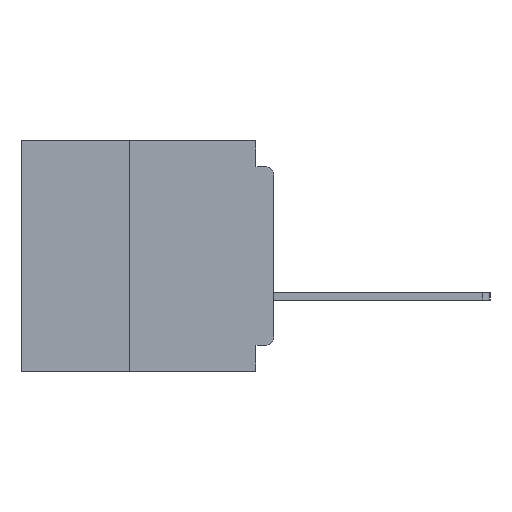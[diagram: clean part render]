
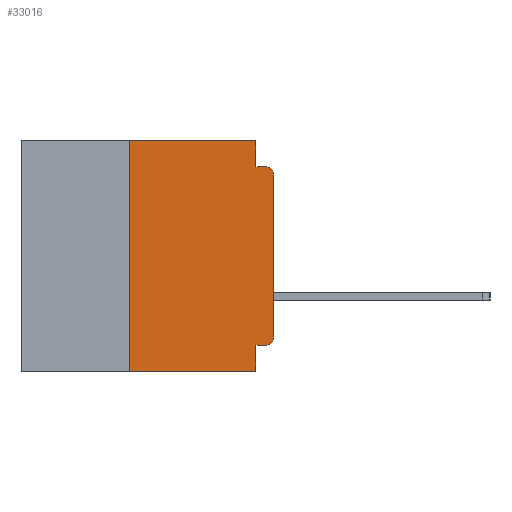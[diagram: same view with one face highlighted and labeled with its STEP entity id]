
A CAD part, left-side view. The second image highlights one B-rep face of the part: STEP entity #33016.
In plain terms, the highlighted planar face has unit normal (-1, 0, 0).
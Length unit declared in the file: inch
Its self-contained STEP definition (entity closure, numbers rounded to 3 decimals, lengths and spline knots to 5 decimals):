
#188 = LINE ( 'NONE', #37120, #32619 ) ;
#919 = CARTESIAN_POINT ( 'NONE',  ( 0., 0.031, 0. ) ) ;
#1937 = VECTOR ( 'NONE', #15777, 39.37008 ) ;
#7017 = LINE ( 'NONE', #22400, #28068 ) ;
#7413 = AXIS2_PLACEMENT_3D ( 'NONE', #40201, #14982, #44454 ) ;
#8552 = EDGE_CURVE ( 'NONE', #47240, #24752, #188, .T. ) ;
#8770 = DIRECTION ( 'NONE',  ( 0., 0., 1. ) ) ;
#9043 = CARTESIAN_POINT ( 'NONE',  ( 0., 0.25, -0.4 ) ) ;
#9058 = EDGE_CURVE ( 'NONE', #42572, #22171, #28692, .T. ) ;
#9689 = CARTESIAN_POINT ( 'NONE',  ( 0., 0.031, -0.355 ) ) ;
#11108 = ORIENTED_EDGE ( 'NONE', *, *, #8552, .T. ) ;
#11936 = ORIENTED_EDGE ( 'NONE', *, *, #54126, .T. ) ;
#12481 = VERTEX_POINT ( 'NONE', #44329 ) ;
#14232 = VERTEX_POINT ( 'NONE', #9689 ) ;
#14356 = DIRECTION ( 'NONE',  ( 0., -1., 0. ) ) ;
#14437 = DIRECTION ( 'NONE',  ( 0., 1., 0. ) ) ;
#14982 = DIRECTION ( 'NONE',  ( 1., 0., 0. ) ) ;
#15777 = DIRECTION ( 'NONE',  ( 0., -1., 0. ) ) ;
#17053 = VECTOR ( 'NONE', #14356, 39.37008 ) ;
#17242 = VERTEX_POINT ( 'NONE', #43105 ) ;
#17258 = CARTESIAN_POINT ( 'NONE',  ( 0., 0.015, -0.34 ) ) ;
#17575 = VECTOR ( 'NONE', #42715, 39.37008 ) ;
#18249 = DIRECTION ( 'NONE',  ( -1., 0., 0. ) ) ;
#18378 = CIRCLE ( 'NONE', #29910, 0.015 ) ;
#19150 = EDGE_CURVE ( 'NONE', #28937, #14232, #38069, .T. ) ;
#19928 = LINE ( 'NONE', #46576, #41058 ) ;
#21380 = EDGE_CURVE ( 'NONE', #14232, #12481, #7017, .T. ) ;
#21450 = DIRECTION ( 'NONE',  ( 0., 0., -1. ) ) ;
#22171 = VERTEX_POINT ( 'NONE', #53320 ) ;
#22198 = CARTESIAN_POINT ( 'NONE',  ( 0., 0., -0.34 ) ) ;
#22400 = CARTESIAN_POINT ( 'NONE',  ( 0., 0.031, -0.4 ) ) ;
#24056 = CARTESIAN_POINT ( 'NONE',  ( 0., 0.015, -0.045 ) ) ;
#24752 = VERTEX_POINT ( 'NONE', #25092 ) ;
#25092 = CARTESIAN_POINT ( 'NONE',  ( 0., 0., -0.06 ) ) ;
#25450 = VERTEX_POINT ( 'NONE', #9043 ) ;
#25738 = CIRCLE ( 'NONE', #34081, 0.015 ) ;
#26362 = ORIENTED_EDGE ( 'NONE', *, *, #49178, .F. ) ;
#27010 = EDGE_CURVE ( 'NONE', #25450, #12481, #27399, .T. ) ;
#27398 = VECTOR ( 'NONE', #36341, 39.37008 ) ;
#27399 = LINE ( 'NONE', #34395, #17575 ) ;
#27831 = CARTESIAN_POINT ( 'NONE',  ( 0., 0.031, 0. ) ) ;
#28068 = VECTOR ( 'NONE', #30875, 39.37008 ) ;
#28692 = LINE ( 'NONE', #27831, #27398 ) ;
#28937 = VERTEX_POINT ( 'NONE', #51762 ) ;
#29667 = EDGE_CURVE ( 'NONE', #28937, #47240, #25738, .T. ) ;
#29910 = AXIS2_PLACEMENT_3D ( 'NONE', #43495, #18249, #47762 ) ;
#30875 = DIRECTION ( 'NONE',  ( 0., 0., -1. ) ) ;
#32619 = VECTOR ( 'NONE', #53973, 39.37008 ) ;
#33016 = ADVANCED_FACE ( 'NONE', ( #48007 ), #35936, .F. ) ;
#33030 = LINE ( 'NONE', #41017, #1937 ) ;
#33533 = ORIENTED_EDGE ( 'NONE', *, *, #9058, .F. ) ;
#34081 = AXIS2_PLACEMENT_3D ( 'NONE', #17258, #46761, #21450 ) ;
#34160 = LINE ( 'NONE', #52342, #17053 ) ;
#34395 = CARTESIAN_POINT ( 'NONE',  ( 0., 0.437, -0.4 ) ) ;
#35936 = PLANE ( 'NONE',  #7413 ) ;
#36341 = DIRECTION ( 'NONE',  ( 0., 0., -1. ) ) ;
#36355 = VERTEX_POINT ( 'NONE', #24056 ) ;
#36379 = EDGE_LOOP ( 'NONE', ( #11108, #11936, #38645, #33533, #26362, #44519, #38637, #37073, #54459, #45050 ) ) ;
#36732 = VECTOR ( 'NONE', #14437, 39.37008 ) ;
#37073 = ORIENTED_EDGE ( 'NONE', *, *, #21380, .F. ) ;
#37120 = CARTESIAN_POINT ( 'NONE',  ( 0., 0., 0. ) ) ;
#38069 = LINE ( 'NONE', #39832, #36732 ) ;
#38637 = ORIENTED_EDGE ( 'NONE', *, *, #27010, .T. ) ;
#38645 = ORIENTED_EDGE ( 'NONE', *, *, #47443, .F. ) ;
#39832 = CARTESIAN_POINT ( 'NONE',  ( 0., 0., -0.355 ) ) ;
#40201 = CARTESIAN_POINT ( 'NONE',  ( 0., 0.437, 0. ) ) ;
#41017 = CARTESIAN_POINT ( 'NONE',  ( 0., 0., -0.045 ) ) ;
#41058 = VECTOR ( 'NONE', #8770, 39.37008 ) ;
#42572 = VERTEX_POINT ( 'NONE', #919 ) ;
#42715 = DIRECTION ( 'NONE',  ( 0., -1., 0. ) ) ;
#43105 = CARTESIAN_POINT ( 'NONE',  ( 0., 0.25, 0. ) ) ;
#43495 = CARTESIAN_POINT ( 'NONE',  ( 0., 0.015, -0.06 ) ) ;
#44033 = EDGE_CURVE ( 'NONE', #25450, #17242, #19928, .T. ) ;
#44329 = CARTESIAN_POINT ( 'NONE',  ( 0., 0.031, -0.4 ) ) ;
#44454 = DIRECTION ( 'NONE',  ( 0., 0., -1. ) ) ;
#44519 = ORIENTED_EDGE ( 'NONE', *, *, #44033, .F. ) ;
#45050 = ORIENTED_EDGE ( 'NONE', *, *, #29667, .T. ) ;
#46576 = CARTESIAN_POINT ( 'NONE',  ( 0., 0.25, -0.4 ) ) ;
#46761 = DIRECTION ( 'NONE',  ( -1., 0., 0. ) ) ;
#47240 = VERTEX_POINT ( 'NONE', #22198 ) ;
#47443 = EDGE_CURVE ( 'NONE', #22171, #36355, #33030, .T. ) ;
#47762 = DIRECTION ( 'NONE',  ( 0., 0., -1. ) ) ;
#48007 = FACE_OUTER_BOUND ( 'NONE', #36379, .T. ) ;
#49178 = EDGE_CURVE ( 'NONE', #17242, #42572, #34160, .T. ) ;
#51762 = CARTESIAN_POINT ( 'NONE',  ( 0., 0.015, -0.355 ) ) ;
#52342 = CARTESIAN_POINT ( 'NONE',  ( 0., 0.437, 0. ) ) ;
#53320 = CARTESIAN_POINT ( 'NONE',  ( 0., 0.031, -0.045 ) ) ;
#53973 = DIRECTION ( 'NONE',  ( 0., 0., 1. ) ) ;
#54126 = EDGE_CURVE ( 'NONE', #24752, #36355, #18378, .T. ) ;
#54459 = ORIENTED_EDGE ( 'NONE', *, *, #19150, .F. ) ;
